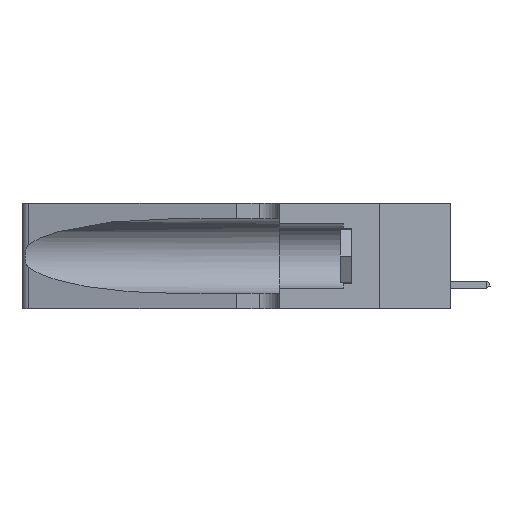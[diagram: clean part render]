
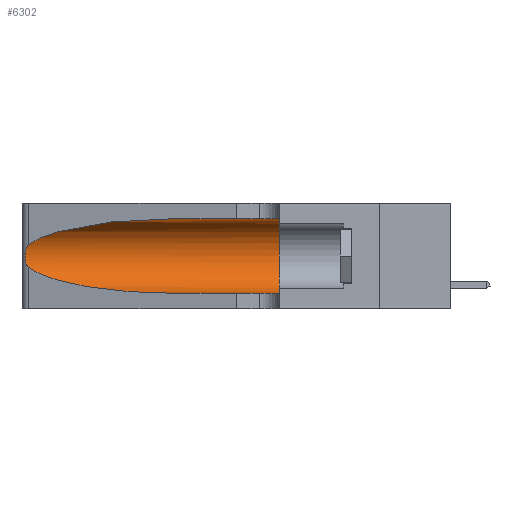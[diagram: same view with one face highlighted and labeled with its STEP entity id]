
A CAD part, left-side view. The second image highlights one B-rep face of the part: STEP entity #6302.
In plain terms, the highlighted cylindrical face has radius 3.308 mm (diameter 6.617 mm), a partial arc.
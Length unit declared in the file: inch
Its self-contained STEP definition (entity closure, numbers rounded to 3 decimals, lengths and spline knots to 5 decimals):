
#1026 = CARTESIAN_POINT ( 'NONE',  ( 0.25555, 1.22994, 0.2215 ) ) ;
#1560 = LINE ( 'NONE', #17640, #23907 ) ;
#1898 = CARTESIAN_POINT ( 'NONE',  ( 0.25487, 1.22718, 0.14631 ) ) ;
#1958 = LINE ( 'NONE', #6746, #18941 ) ;
#1989 = CARTESIAN_POINT ( 'NONE',  ( 0.25487, 1.22718, 0.22369 ) ) ;
#2872 = VERTEX_POINT ( 'NONE', #16788 ) ;
#3291 = CARTESIAN_POINT ( 'NONE',  ( 0.1305, 1.61858, 0.185 ) ) ;
#3528 = CARTESIAN_POINT ( 'NONE',  ( 0.25639, 1.23184, 0.21858 ) ) ;
#4180 = CARTESIAN_POINT ( 'NONE',  ( 0.25555, 1.22993, 0.14849 ) ) ;
#4458 = EDGE_CURVE ( 'NONE', #6383, #12773, #27012, .T. ) ;
#5441 = ORIENTED_EDGE ( 'NONE', *, *, #28555, .T. ) ;
#6302 = ADVANCED_FACE ( 'NONE', ( #21217 ), #21962, .F. ) ;
#6383 = VERTEX_POINT ( 'NONE', #17137 ) ;
#6406 = CARTESIAN_POINT ( 'NONE',  ( 0.25789, 1.23486, 0.15765 ) ) ;
#6544 = CARTESIAN_POINT ( 'NONE',  ( 0.2373, 1.15595, 0.28018 ) ) ;
#6555 = ORIENTED_EDGE ( 'NONE', *, *, #10389, .T. ) ;
#6587 = DIRECTION ( 'NONE',  ( 0., -1., 0. ) ) ;
#6746 = CARTESIAN_POINT ( 'NONE',  ( 0.1305, 1.61858, 0.31525 ) ) ;
#6941 = ORIENTED_EDGE ( 'NONE', *, *, #8884, .T. ) ;
#7027 = CARTESIAN_POINT ( 'NONE',  ( 0.1305, 0.72297, 0.05475 ) ) ;
#7439 = CARTESIAN_POINT ( 'NONE',  ( 0.1305, 0.72297, 0.05475 ) ) ;
#8884 = EDGE_CURVE ( 'NONE', #2872, #9077, #28447, .T. ) ;
#8910 = CARTESIAN_POINT ( 'NONE',  ( 0.1305, 0.72297, 0.31525 ) ) ;
#9029 = CARTESIAN_POINT ( 'NONE',  ( 0.18966, 0.96281, 0.31525 ) ) ;
#9077 = VERTEX_POINT ( 'NONE', #7439 ) ;
#9214 = CARTESIAN_POINT ( 'NONE',  ( 0.25639, 1.23186, 0.15144 ) ) ;
#9295 = CARTESIAN_POINT ( 'NONE',  ( 0.18966, 0.96281, 0.05475 ) ) ;
#9312 = CARTESIAN_POINT ( 'NONE',  ( 0.1305, 0.72297, 0.31525 ) ) ;
#10389 = EDGE_CURVE ( 'NONE', #29617, #26716, #20807, .T. ) ;
#12773 = VERTEX_POINT ( 'NONE', #23791 ) ;
#13007 = EDGE_CURVE ( 'NONE', #26716, #2872, #18012, .T. ) ;
#14099 = CARTESIAN_POINT ( 'NONE',  ( 0.25854, 1.2359, 0.20912 ) ) ;
#14212 = CARTESIAN_POINT ( 'NONE',  ( 0.26017, 1.23833, 0.17102 ) ) ;
#16150 = CARTESIAN_POINT ( 'NONE',  ( 0.25787, 1.23484, 0.2124 ) ) ;
#16643 = EDGE_CURVE ( 'NONE', #29617, #6383, #1958, .T. ) ;
#16788 = CARTESIAN_POINT ( 'NONE',  ( 0.25487, 1.22718, 0.14631 ) ) ;
#17137 = CARTESIAN_POINT ( 'NONE',  ( 0.1305, 0.35, 0.31525 ) ) ;
#17589 = AXIS2_PLACEMENT_3D ( 'NONE', #20414, #18667, #21260 ) ;
#17640 = CARTESIAN_POINT ( 'NONE',  ( 0.1305, 1.61858, 0.05475 ) ) ;
#18012 = B_SPLINE_CURVE_WITH_KNOTS ( 'NONE', 3,
 ( #23146, #1026, #3528, #16150, #14099, #18739, #26143, #18842, #14212, #28744, #6406, #9214, #4180, #26469 ),
 .UNSPECIFIED., .F., .F.,
 ( 4, 2, 2, 2, 2, 2, 4 ),
 ( 0., 0.00027, 0.00053, 0.00107, 0.0016, 0.00187, 0.00214 ),
 .UNSPECIFIED. ) ;
#18667 = DIRECTION ( 'NONE',  ( 0., 1., 0. ) ) ;
#18739 = CARTESIAN_POINT ( 'NONE',  ( 0.26018, 1.23835, 0.19895 ) ) ;
#18842 = CARTESIAN_POINT ( 'NONE',  ( 0.26075, 1.23896, 0.178 ) ) ;
#18941 = VECTOR ( 'NONE', #31577, 39.37008 ) ;
#20414 = CARTESIAN_POINT ( 'NONE',  ( 0.1305, 0.35, 0.185 ) ) ;
#20807 =( BOUNDED_CURVE ( )  B_SPLINE_CURVE ( 3, ( #8910, #9029, #6544, #1989 ),
 .UNSPECIFIED., .F., .T. ) 
 B_SPLINE_CURVE_WITH_KNOTS ( ( 4, 4 ),
 ( 1.5708, 2.84003 ),
 .UNSPECIFIED. ) 
 CURVE ( )  GEOMETRIC_REPRESENTATION_ITEM ( )  RATIONAL_B_SPLINE_CURVE ( ( 1., 0.87, 0.87, 1. ) ) 
 REPRESENTATION_ITEM ( '' )  );
#21217 = FACE_OUTER_BOUND ( 'NONE', #27632, .T. ) ;
#21260 = DIRECTION ( 'NONE',  ( 0., 0., 1. ) ) ;
#21843 = CARTESIAN_POINT ( 'NONE',  ( 0.2373, 1.15595, 0.08982 ) ) ;
#21962 = CYLINDRICAL_SURFACE ( 'NONE', #29384, 0.13025 ) ;
#23146 = CARTESIAN_POINT ( 'NONE',  ( 0.25487, 1.22718, 0.22369 ) ) ;
#23182 = DIRECTION ( 'NONE',  ( 0., 0., -1. ) ) ;
#23791 = CARTESIAN_POINT ( 'NONE',  ( 0.1305, 0.35, 0.05475 ) ) ;
#23907 = VECTOR ( 'NONE', #29789, 39.37008 ) ;
#25252 = ORIENTED_EDGE ( 'NONE', *, *, #4458, .F. ) ;
#26143 = CARTESIAN_POINT ( 'NONE',  ( 0.26075, 1.23896, 0.19203 ) ) ;
#26469 = CARTESIAN_POINT ( 'NONE',  ( 0.25487, 1.22718, 0.14631 ) ) ;
#26716 = VERTEX_POINT ( 'NONE', #30614 ) ;
#26837 = ORIENTED_EDGE ( 'NONE', *, *, #16643, .F. ) ;
#27012 = CIRCLE ( 'NONE', #17589, 0.13025 ) ;
#27097 = ORIENTED_EDGE ( 'NONE', *, *, #13007, .T. ) ;
#27632 = EDGE_LOOP ( 'NONE', ( #6555, #27097, #6941, #5441, #25252, #26837 ) ) ;
#28447 =( BOUNDED_CURVE ( )  B_SPLINE_CURVE ( 3, ( #1898, #21843, #9295, #7027 ),
 .UNSPECIFIED., .F., .T. ) 
 B_SPLINE_CURVE_WITH_KNOTS ( ( 4, 4 ),
 ( 3.44316, 4.71239 ),
 .UNSPECIFIED. ) 
 CURVE ( )  GEOMETRIC_REPRESENTATION_ITEM ( )  RATIONAL_B_SPLINE_CURVE ( ( 1., 0.87, 0.87, 1. ) ) 
 REPRESENTATION_ITEM ( '' )  );
#28555 = EDGE_CURVE ( 'NONE', #9077, #12773, #1560, .T. ) ;
#28744 = CARTESIAN_POINT ( 'NONE',  ( 0.25856, 1.23593, 0.16098 ) ) ;
#29384 = AXIS2_PLACEMENT_3D ( 'NONE', #3291, #6587, #23182 ) ;
#29617 = VERTEX_POINT ( 'NONE', #9312 ) ;
#29789 = DIRECTION ( 'NONE',  ( 0., -1., 0. ) ) ;
#30614 = CARTESIAN_POINT ( 'NONE',  ( 0.25487, 1.22718, 0.22369 ) ) ;
#31577 = DIRECTION ( 'NONE',  ( 0., -1., 0. ) ) ;
